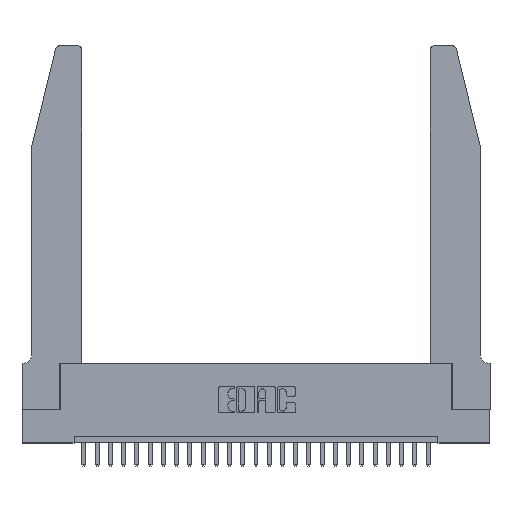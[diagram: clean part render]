
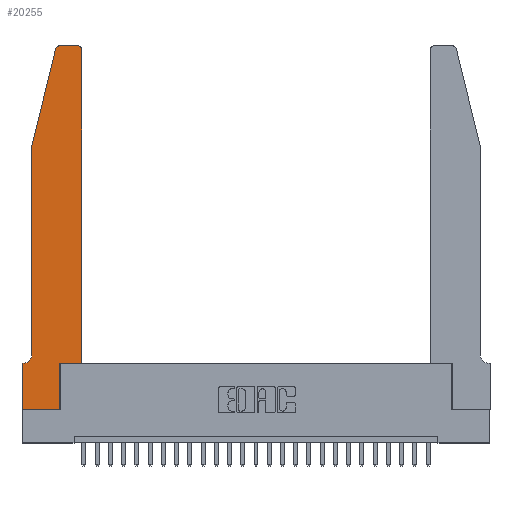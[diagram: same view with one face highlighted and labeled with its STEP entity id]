
A CAD part, top view. The second image highlights one B-rep face of the part: STEP entity #20255.
In plain terms, the highlighted planar face has unit normal (0, 0, 1).
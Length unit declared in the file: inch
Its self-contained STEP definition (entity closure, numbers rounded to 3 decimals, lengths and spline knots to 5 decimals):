
#572 = DIRECTION ( 'NONE',  ( 1., 0., 0. ) ) ;
#620 = DIRECTION ( 'NONE',  ( 1., 0., 0. ) ) ;
#1008 = DIRECTION ( 'NONE',  ( -1., 0., 0. ) ) ;
#1068 = VECTOR ( 'NONE', #620, 39.37008 ) ;
#1496 = ORIENTED_EDGE ( 'NONE', *, *, #16453, .T. ) ;
#2162 = VECTOR ( 'NONE', #16169, 39.37008 ) ;
#2210 = CARTESIAN_POINT ( 'NONE',  ( 0., 0., 0.37 ) ) ;
#2513 = AXIS2_PLACEMENT_3D ( 'NONE', #21797, #17487, #572 ) ;
#3403 = ORIENTED_EDGE ( 'NONE', *, *, #11424, .T. ) ;
#3588 = VECTOR ( 'NONE', #9917, 39.37008 ) ;
#4191 = VERTEX_POINT ( 'NONE', #22343 ) ;
#4389 = LINE ( 'NONE', #15203, #12269 ) ;
#4489 = CARTESIAN_POINT ( 'NONE',  ( 0.2605, 2.75, 0.37 ) ) ;
#4523 = DIRECTION ( 'NONE',  ( 1., 0., 0. ) ) ;
#4816 = ORIENTED_EDGE ( 'NONE', *, *, #21889, .T. ) ;
#4928 = FACE_OUTER_BOUND ( 'NONE', #15066, .T. ) ;
#4979 = DIRECTION ( 'NONE',  ( 0., 0., -1. ) ) ;
#4999 = ORIENTED_EDGE ( 'NONE', *, *, #5439, .T. ) ;
#5439 = EDGE_CURVE ( 'NONE', #11691, #6540, #24484, .T. ) ;
#5451 = PLANE ( 'NONE',  #24892 ) ;
#5651 = CARTESIAN_POINT ( 'NONE',  ( 0., 0., 0.37 ) ) ;
#5690 = CARTESIAN_POINT ( 'NONE',  ( 0.25487, 2.72718, 0.37 ) ) ;
#6540 = VERTEX_POINT ( 'NONE', #17794 ) ;
#6878 = AXIS2_PLACEMENT_3D ( 'NONE', #13598, #4979, #1008 ) ;
#7407 = CARTESIAN_POINT ( 'NONE',  ( 0.2865, 0.35, 0.37 ) ) ;
#7844 = DIRECTION ( 'NONE',  ( 0., -1., 0. ) ) ;
#8114 = LINE ( 'NONE', #26093, #24207 ) ;
#8535 = DIRECTION ( 'NONE',  ( -1., 0., 0. ) ) ;
#8949 = CARTESIAN_POINT ( 'NONE',  ( 0., 0.35, 0.37 ) ) ;
#9119 = VECTOR ( 'NONE', #21852, 39.37008 ) ;
#9467 = EDGE_CURVE ( 'NONE', #19673, #10049, #13384, .T. ) ;
#9618 = LINE ( 'NONE', #2210, #1068 ) ;
#9837 = VERTEX_POINT ( 'NONE', #20611 ) ;
#9847 = CIRCLE ( 'NONE', #2513, 0.03 ) ;
#9917 = DIRECTION ( 'NONE',  ( 0., 1., 0. ) ) ;
#10002 = ORIENTED_EDGE ( 'NONE', *, *, #15561, .T. ) ;
#10049 = VERTEX_POINT ( 'NONE', #7407 ) ;
#11014 = ORIENTED_EDGE ( 'NONE', *, *, #20052, .T. ) ;
#11041 = ORIENTED_EDGE ( 'NONE', *, *, #24477, .T. ) ;
#11353 = DIRECTION ( 'NONE',  ( 0., -1., 0. ) ) ;
#11359 = VERTEX_POINT ( 'NONE', #20237 ) ;
#11422 = VECTOR ( 'NONE', #13000, 39.37008 ) ;
#11424 = EDGE_CURVE ( 'NONE', #10049, #4191, #26112, .T. ) ;
#11691 = VERTEX_POINT ( 'NONE', #17892 ) ;
#11844 = CARTESIAN_POINT ( 'NONE',  ( 0.2865, 0., 0.37 ) ) ;
#11978 = LINE ( 'NONE', #4489, #15892 ) ;
#12159 = CARTESIAN_POINT ( 'NONE',  ( 0.4505, 0.35, 0.37 ) ) ;
#12269 = VECTOR ( 'NONE', #11353, 39.37008 ) ;
#12432 = VERTEX_POINT ( 'NONE', #18589 ) ;
#12939 = AXIS2_PLACEMENT_3D ( 'NONE', #19118, #17182, #4523 ) ;
#13000 = DIRECTION ( 'NONE',  ( -1., 0., 0. ) ) ;
#13030 = VERTEX_POINT ( 'NONE', #8949 ) ;
#13217 = VECTOR ( 'NONE', #7844, 39.37008 ) ;
#13384 = LINE ( 'NONE', #19921, #9119 ) ;
#13598 = CARTESIAN_POINT ( 'NONE',  ( 0.0055, 0.42, 0.37 ) ) ;
#13688 = LINE ( 'NONE', #17573, #11422 ) ;
#13801 = DIRECTION ( 'NONE',  ( -0.239, -0.971, 0. ) ) ;
#15066 = EDGE_LOOP ( 'NONE', ( #20837, #11014, #15337, #10002, #1496, #4816, #11041, #22195, #21159, #3403, #24742, #4999 ) ) ;
#15073 = LINE ( 'NONE', #18257, #3588 ) ;
#15203 = CARTESIAN_POINT ( 'NONE',  ( 0.0755, 2., 0.37 ) ) ;
#15337 = ORIENTED_EDGE ( 'NONE', *, *, #21966, .T. ) ;
#15430 = EDGE_CURVE ( 'NONE', #23241, #19673, #9618, .T. ) ;
#15500 = CARTESIAN_POINT ( 'NONE',  ( 0., 0., 0.37 ) ) ;
#15561 = EDGE_CURVE ( 'NONE', #12432, #9837, #4389, .T. ) ;
#15892 = VECTOR ( 'NONE', #8535, 39.37008 ) ;
#16169 = DIRECTION ( 'NONE',  ( 1., 0., 0. ) ) ;
#16453 = EDGE_CURVE ( 'NONE', #9837, #26606, #24695, .T. ) ;
#17182 = DIRECTION ( 'NONE',  ( 0., 0., 1. ) ) ;
#17487 = DIRECTION ( 'NONE',  ( 0., 0., 1. ) ) ;
#17573 = CARTESIAN_POINT ( 'NONE',  ( 0.0755, 0.35, 0.37 ) ) ;
#17794 = CARTESIAN_POINT ( 'NONE',  ( 0.4205, 2.75, 0.37 ) ) ;
#17892 = CARTESIAN_POINT ( 'NONE',  ( 0.4505, 2.72, 0.37 ) ) ;
#18257 = CARTESIAN_POINT ( 'NONE',  ( 0.4505, 0.35, 0.37 ) ) ;
#18589 = CARTESIAN_POINT ( 'NONE',  ( 0.0755, 2., 0.37 ) ) ;
#19118 = CARTESIAN_POINT ( 'NONE',  ( 0.4205, 2.72, 0.37 ) ) ;
#19673 = VERTEX_POINT ( 'NONE', #11844 ) ;
#19921 = CARTESIAN_POINT ( 'NONE',  ( 0.2865, 0.35, 0.37 ) ) ;
#20052 = EDGE_CURVE ( 'NONE', #11359, #25211, #9847, .T. ) ;
#20237 = CARTESIAN_POINT ( 'NONE',  ( 0.284, 2.75, 0.37 ) ) ;
#20255 = ADVANCED_FACE ( 'NONE', ( #4928 ), #5451, .T. ) ;
#20611 = CARTESIAN_POINT ( 'NONE',  ( 0.0755, 0.42, 0.37 ) ) ;
#20837 = ORIENTED_EDGE ( 'NONE', *, *, #23681, .T. ) ;
#20959 = EDGE_CURVE ( 'NONE', #4191, #11691, #15073, .T. ) ;
#21159 = ORIENTED_EDGE ( 'NONE', *, *, #9467, .T. ) ;
#21441 = LINE ( 'NONE', #5651, #13217 ) ;
#21485 = CARTESIAN_POINT ( 'NONE',  ( 0.0055, 0.35, 0.37 ) ) ;
#21797 = CARTESIAN_POINT ( 'NONE',  ( 0.284, 2.72, 0.37 ) ) ;
#21852 = DIRECTION ( 'NONE',  ( 0., 1., 0. ) ) ;
#21889 = EDGE_CURVE ( 'NONE', #26606, #13030, #13688, .T. ) ;
#21966 = EDGE_CURVE ( 'NONE', #25211, #12432, #8114, .T. ) ;
#22195 = ORIENTED_EDGE ( 'NONE', *, *, #15430, .T. ) ;
#22343 = CARTESIAN_POINT ( 'NONE',  ( 0.4505, 0.35, 0.37 ) ) ;
#23241 = VERTEX_POINT ( 'NONE', #15500 ) ;
#23681 = EDGE_CURVE ( 'NONE', #6540, #11359, #11978, .T. ) ;
#24207 = VECTOR ( 'NONE', #13801, 39.37008 ) ;
#24279 = CARTESIAN_POINT ( 'NONE',  ( 0., 0.35, 0.37 ) ) ;
#24367 = DIRECTION ( 'NONE',  ( 0., 0., 1. ) ) ;
#24477 = EDGE_CURVE ( 'NONE', #13030, #23241, #21441, .T. ) ;
#24484 = CIRCLE ( 'NONE', #12939, 0.03 ) ;
#24695 = CIRCLE ( 'NONE', #6878, 0.07 ) ;
#24742 = ORIENTED_EDGE ( 'NONE', *, *, #20959, .T. ) ;
#24892 = AXIS2_PLACEMENT_3D ( 'NONE', #24279, #24367, #26364 ) ;
#25211 = VERTEX_POINT ( 'NONE', #5690 ) ;
#26093 = CARTESIAN_POINT ( 'NONE',  ( 0.0755, 2., 0.37 ) ) ;
#26112 = LINE ( 'NONE', #12159, #2162 ) ;
#26364 = DIRECTION ( 'NONE',  ( 1., 0., 0. ) ) ;
#26606 = VERTEX_POINT ( 'NONE', #21485 ) ;
